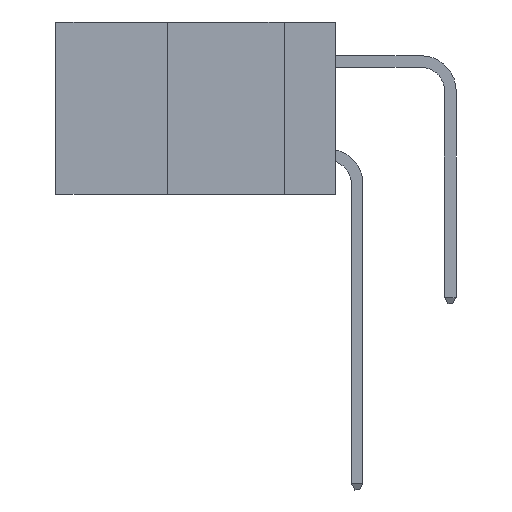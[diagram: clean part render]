
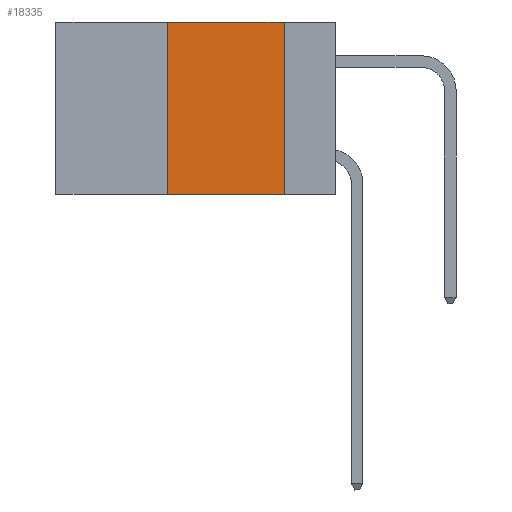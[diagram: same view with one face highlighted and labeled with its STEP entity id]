
A CAD part, left-side view. The second image highlights one B-rep face of the part: STEP entity #18335.
In plain terms, the highlighted planar face has unit normal (-1, 0, 0).
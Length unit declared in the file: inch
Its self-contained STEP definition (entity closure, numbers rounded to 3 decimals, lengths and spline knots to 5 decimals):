
#867 = LINE ( 'NONE', #10563, #5923 ) ;
#974 = VECTOR ( 'NONE', #18404, 39.37008 ) ;
#1786 = AXIS2_PLACEMENT_3D ( 'NONE', #17722, #15913, #4670 ) ;
#2132 = EDGE_CURVE ( 'NONE', #23737, #11587, #21058, .T. ) ;
#3410 = EDGE_CURVE ( 'NONE', #19786, #6007, #10435, .T. ) ;
#4588 = EDGE_LOOP ( 'NONE', ( #11436, #18216, #7592, #22008 ) ) ;
#4670 = DIRECTION ( 'NONE',  ( 0., 0., -1. ) ) ;
#5923 = VECTOR ( 'NONE', #23599, 39.37008 ) ;
#6007 = VERTEX_POINT ( 'NONE', #23935 ) ;
#6663 = VECTOR ( 'NONE', #21783, 39.37008 ) ;
#7592 = ORIENTED_EDGE ( 'NONE', *, *, #2132, .F. ) ;
#8818 = CARTESIAN_POINT ( 'NONE',  ( 0., 0.36, -0.37 ) ) ;
#10435 = LINE ( 'NONE', #16520, #974 ) ;
#10563 = CARTESIAN_POINT ( 'NONE',  ( 0., 0.6, 0. ) ) ;
#10565 = CARTESIAN_POINT ( 'NONE',  ( 0., 0.36, 0. ) ) ;
#11436 = ORIENTED_EDGE ( 'NONE', *, *, #3410, .F. ) ;
#11587 = VERTEX_POINT ( 'NONE', #23154 ) ;
#12124 = PLANE ( 'NONE',  #1786 ) ;
#14061 = CARTESIAN_POINT ( 'NONE',  ( 0., 0.6, -0.37 ) ) ;
#15913 = DIRECTION ( 'NONE',  ( 1., 0., 0. ) ) ;
#15968 = DIRECTION ( 'NONE',  ( 0., -1., 0. ) ) ;
#16520 = CARTESIAN_POINT ( 'NONE',  ( 0., 0.11, 0. ) ) ;
#16534 = CARTESIAN_POINT ( 'NONE',  ( 0., 0.11, 0. ) ) ;
#17722 = CARTESIAN_POINT ( 'NONE',  ( 0., 0.6, 0. ) ) ;
#18216 = ORIENTED_EDGE ( 'NONE', *, *, #23665, .F. ) ;
#18335 = ADVANCED_FACE ( 'NONE', ( #20525 ), #12124, .F. ) ;
#18404 = DIRECTION ( 'NONE',  ( 0., 0., -1. ) ) ;
#19006 = EDGE_CURVE ( 'NONE', #23737, #6007, #20774, .T. ) ;
#19597 = VECTOR ( 'NONE', #15968, 39.37008 ) ;
#19786 = VERTEX_POINT ( 'NONE', #16534 ) ;
#20525 = FACE_OUTER_BOUND ( 'NONE', #4588, .T. ) ;
#20774 = LINE ( 'NONE', #14061, #19597 ) ;
#21058 = LINE ( 'NONE', #10565, #6663 ) ;
#21783 = DIRECTION ( 'NONE',  ( 0., 0., 1. ) ) ;
#22008 = ORIENTED_EDGE ( 'NONE', *, *, #19006, .T. ) ;
#23154 = CARTESIAN_POINT ( 'NONE',  ( 0., 0.36, 0. ) ) ;
#23599 = DIRECTION ( 'NONE',  ( 0., -1., 0. ) ) ;
#23665 = EDGE_CURVE ( 'NONE', #11587, #19786, #867, .T. ) ;
#23737 = VERTEX_POINT ( 'NONE', #8818 ) ;
#23935 = CARTESIAN_POINT ( 'NONE',  ( 0., 0.11, -0.37 ) ) ;
